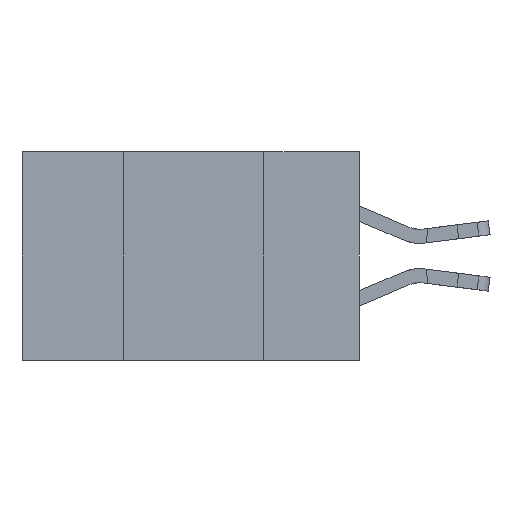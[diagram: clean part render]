
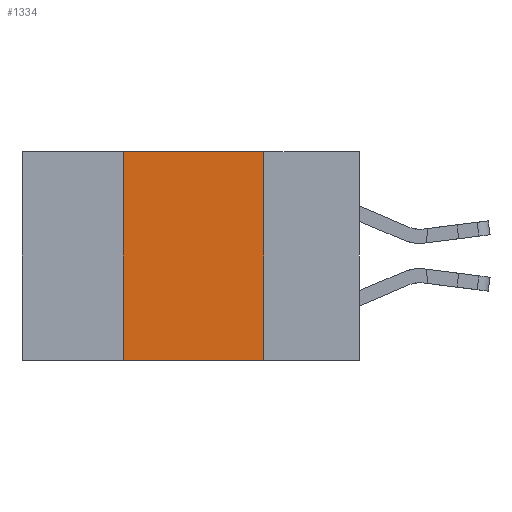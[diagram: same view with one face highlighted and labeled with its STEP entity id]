
A CAD part, left-side view. The second image highlights one B-rep face of the part: STEP entity #1334.
In plain terms, the highlighted planar face has unit normal (-1, 0, 0).
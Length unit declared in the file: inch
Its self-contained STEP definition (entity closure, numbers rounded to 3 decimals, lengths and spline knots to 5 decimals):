
#21 = CARTESIAN_POINT ( 'NONE',  ( 0., 0.42, 0. ) ) ;
#572 = EDGE_CURVE ( 'NONE', #18626, #9854, #18591, .T. ) ;
#1040 = VECTOR ( 'NONE', #11654, 39.37008 ) ;
#1160 = CARTESIAN_POINT ( 'NONE',  ( 0., 0.17, 0. ) ) ;
#1191 = EDGE_LOOP ( 'NONE', ( #10166, #18413, #19775, #13058 ) ) ;
#1334 = ADVANCED_FACE ( 'NONE', ( #2390 ), #4672, .F. ) ;
#2390 = FACE_OUTER_BOUND ( 'NONE', #1191, .T. ) ;
#4672 = PLANE ( 'NONE',  #19824 ) ;
#6831 = DIRECTION ( 'NONE',  ( 0., 0., 1. ) ) ;
#7644 = DIRECTION ( 'NONE',  ( 0., 0., -1. ) ) ;
#7720 = VERTEX_POINT ( 'NONE', #17497 ) ;
#8941 = LINE ( 'NONE', #16421, #1040 ) ;
#9223 = DIRECTION ( 'NONE',  ( 0., 0., -1. ) ) ;
#9416 = DIRECTION ( 'NONE',  ( 1., 0., 0. ) ) ;
#9854 = VERTEX_POINT ( 'NONE', #1160 ) ;
#9883 = CARTESIAN_POINT ( 'NONE',  ( 0., 0.42, 0. ) ) ;
#10166 = ORIENTED_EDGE ( 'NONE', *, *, #14038, .F. ) ;
#10892 = CARTESIAN_POINT ( 'NONE',  ( 0., 0.6, 0. ) ) ;
#11387 = VECTOR ( 'NONE', #6831, 39.37008 ) ;
#11654 = DIRECTION ( 'NONE',  ( 0., -1., 0. ) ) ;
#12264 = LINE ( 'NONE', #18911, #17349 ) ;
#13058 = ORIENTED_EDGE ( 'NONE', *, *, #17655, .T. ) ;
#14038 = EDGE_CURVE ( 'NONE', #9854, #19882, #12264, .T. ) ;
#15779 = CARTESIAN_POINT ( 'NONE',  ( 0., 0.6, 0. ) ) ;
#15919 = CARTESIAN_POINT ( 'NONE',  ( 0., 0.17, -0.37 ) ) ;
#16421 = CARTESIAN_POINT ( 'NONE',  ( 0., 0.6, -0.37 ) ) ;
#17349 = VECTOR ( 'NONE', #9223, 39.37008 ) ;
#17497 = CARTESIAN_POINT ( 'NONE',  ( 0., 0.42, -0.37 ) ) ;
#17619 = EDGE_CURVE ( 'NONE', #7720, #18626, #18694, .T. ) ;
#17655 = EDGE_CURVE ( 'NONE', #7720, #19882, #8941, .T. ) ;
#18260 = DIRECTION ( 'NONE',  ( 0., -1., 0. ) ) ;
#18413 = ORIENTED_EDGE ( 'NONE', *, *, #572, .F. ) ;
#18591 = LINE ( 'NONE', #10892, #20318 ) ;
#18626 = VERTEX_POINT ( 'NONE', #21 ) ;
#18694 = LINE ( 'NONE', #9883, #11387 ) ;
#18911 = CARTESIAN_POINT ( 'NONE',  ( 0., 0.17, 0. ) ) ;
#19775 = ORIENTED_EDGE ( 'NONE', *, *, #17619, .F. ) ;
#19824 = AXIS2_PLACEMENT_3D ( 'NONE', #15779, #9416, #7644 ) ;
#19882 = VERTEX_POINT ( 'NONE', #15919 ) ;
#20318 = VECTOR ( 'NONE', #18260, 39.37008 ) ;
